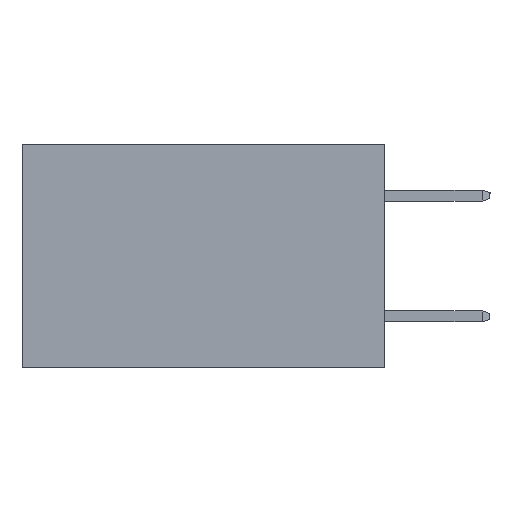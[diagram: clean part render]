
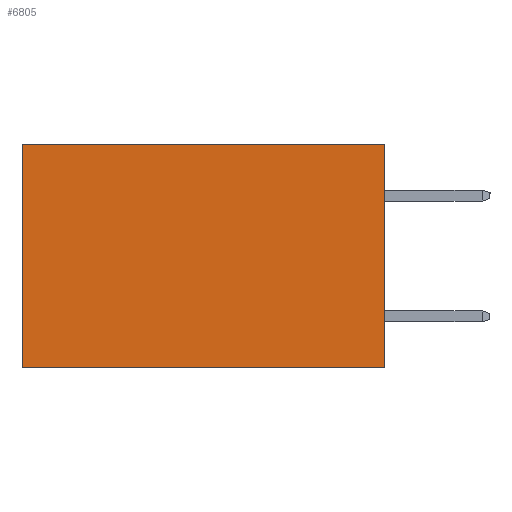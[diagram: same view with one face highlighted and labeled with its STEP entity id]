
A CAD part, left-side view. The second image highlights one B-rep face of the part: STEP entity #6805.
In plain terms, the highlighted planar face has unit normal (-1, 0, 0).
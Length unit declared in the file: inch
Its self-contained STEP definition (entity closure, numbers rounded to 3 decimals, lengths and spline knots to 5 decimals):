
#172 = EDGE_CURVE ( 'NONE', #11151, #2007, #7407, .T. ) ;
#673 = VERTEX_POINT ( 'NONE', #3495 ) ;
#698 = DIRECTION ( 'NONE',  ( 0., 0., -1. ) ) ;
#969 = LINE ( 'NONE', #9693, #5679 ) ;
#1404 = CARTESIAN_POINT ( 'NONE',  ( 0.2615, 0.6, -0.37 ) ) ;
#1651 = CARTESIAN_POINT ( 'NONE',  ( 0.2615, 0., -0.37 ) ) ;
#1844 = VECTOR ( 'NONE', #698, 39.37008 ) ;
#2007 = VERTEX_POINT ( 'NONE', #8293 ) ;
#2354 = CARTESIAN_POINT ( 'NONE',  ( 0.2615, 0., 0. ) ) ;
#3365 = DIRECTION ( 'NONE',  ( 0., 0., -1. ) ) ;
#3452 = DIRECTION ( 'NONE',  ( 0., 0., -1. ) ) ;
#3495 = CARTESIAN_POINT ( 'NONE',  ( 0.2615, 0.6, 0. ) ) ;
#4080 = CARTESIAN_POINT ( 'NONE',  ( 0.2615, 0., 0. ) ) ;
#4689 = ORIENTED_EDGE ( 'NONE', *, *, #172, .F. ) ;
#5679 = VECTOR ( 'NONE', #8675, 39.37008 ) ;
#6388 = ORIENTED_EDGE ( 'NONE', *, *, #9169, .T. ) ;
#6465 = CARTESIAN_POINT ( 'NONE',  ( 0.2615, 0.6, -0.37 ) ) ;
#6671 = LINE ( 'NONE', #2354, #6688 ) ;
#6688 = VECTOR ( 'NONE', #11849, 39.37008 ) ;
#6805 = ADVANCED_FACE ( 'NONE', ( #11065 ), #10110, .F. ) ;
#7407 = LINE ( 'NONE', #1651, #1844 ) ;
#8043 = EDGE_CURVE ( 'NONE', #2007, #8171, #969, .T. ) ;
#8171 = VERTEX_POINT ( 'NONE', #6465 ) ;
#8293 = CARTESIAN_POINT ( 'NONE',  ( 0.2615, 0., -0.37 ) ) ;
#8675 = DIRECTION ( 'NONE',  ( 0., 1., 0. ) ) ;
#9138 = DIRECTION ( 'NONE',  ( 1., 0., 0. ) ) ;
#9169 = EDGE_CURVE ( 'NONE', #11151, #673, #6671, .T. ) ;
#9278 = EDGE_CURVE ( 'NONE', #673, #8171, #11983, .T. ) ;
#9690 = ORIENTED_EDGE ( 'NONE', *, *, #8043, .F. ) ;
#9693 = CARTESIAN_POINT ( 'NONE',  ( 0.2615, 0., -0.37 ) ) ;
#9716 = VECTOR ( 'NONE', #3365, 39.37008 ) ;
#10110 = PLANE ( 'NONE',  #11699 ) ;
#10784 = EDGE_LOOP ( 'NONE', ( #12212, #9690, #4689, #6388 ) ) ;
#11065 = FACE_OUTER_BOUND ( 'NONE', #10784, .T. ) ;
#11151 = VERTEX_POINT ( 'NONE', #4080 ) ;
#11264 = CARTESIAN_POINT ( 'NONE',  ( 0.2615, 0., -0.37 ) ) ;
#11699 = AXIS2_PLACEMENT_3D ( 'NONE', #11264, #9138, #3452 ) ;
#11849 = DIRECTION ( 'NONE',  ( 0., 1., 0. ) ) ;
#11983 = LINE ( 'NONE', #1404, #9716 ) ;
#12212 = ORIENTED_EDGE ( 'NONE', *, *, #9278, .T. ) ;
